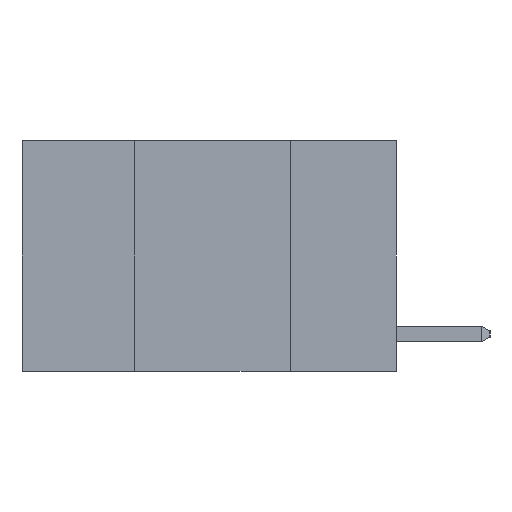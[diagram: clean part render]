
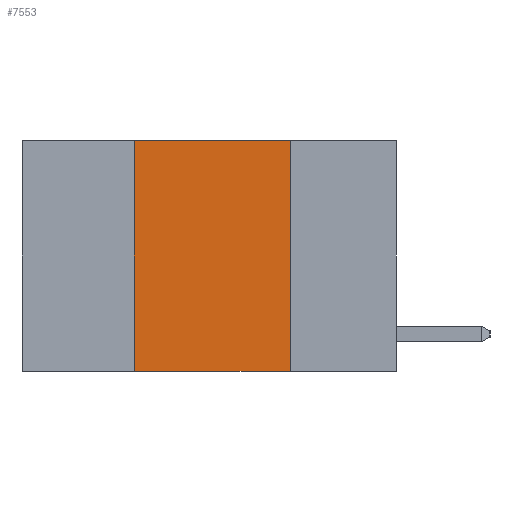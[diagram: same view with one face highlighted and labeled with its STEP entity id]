
A CAD part, left-side view. The second image highlights one B-rep face of the part: STEP entity #7553.
In plain terms, the highlighted planar face has unit normal (-1, 0, 0).
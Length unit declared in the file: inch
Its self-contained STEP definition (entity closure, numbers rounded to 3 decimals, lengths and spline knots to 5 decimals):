
#228 = VECTOR ( 'NONE', #649, 39.37008 ) ;
#649 = DIRECTION ( 'NONE',  ( 0., 0., -1. ) ) ;
#696 = DIRECTION ( 'NONE',  ( 0., 0., 1. ) ) ;
#790 = CARTESIAN_POINT ( 'NONE',  ( 0., 0.42, -0.37 ) ) ;
#941 = ORIENTED_EDGE ( 'NONE', *, *, #4402, .F. ) ;
#1168 = ORIENTED_EDGE ( 'NONE', *, *, #5838, .T. ) ;
#1659 = DIRECTION ( 'NONE',  ( 1., 0., 0. ) ) ;
#1970 = VERTEX_POINT ( 'NONE', #790 ) ;
#2298 = CARTESIAN_POINT ( 'NONE',  ( 0., 0.6, 0. ) ) ;
#2876 = ORIENTED_EDGE ( 'NONE', *, *, #8790, .F. ) ;
#2977 = DIRECTION ( 'NONE',  ( 0., -1., 0. ) ) ;
#3306 = CARTESIAN_POINT ( 'NONE',  ( 0., 0.42, 0. ) ) ;
#3360 = CARTESIAN_POINT ( 'NONE',  ( 0., 0.6, -0.37 ) ) ;
#3532 = CARTESIAN_POINT ( 'NONE',  ( 0., 0.17, 0. ) ) ;
#3566 = CARTESIAN_POINT ( 'NONE',  ( 0., 0.17, 0. ) ) ;
#3601 = VERTEX_POINT ( 'NONE', #3306 ) ;
#3860 = AXIS2_PLACEMENT_3D ( 'NONE', #5247, #1659, #6665 ) ;
#4402 = EDGE_CURVE ( 'NONE', #6031, #7622, #7837, .T. ) ;
#4522 = PLANE ( 'NONE',  #3860 ) ;
#4863 = EDGE_CURVE ( 'NONE', #1970, #3601, #8995, .T. ) ;
#5247 = CARTESIAN_POINT ( 'NONE',  ( 0., 0.6, 0. ) ) ;
#5514 = DIRECTION ( 'NONE',  ( 0., -1., 0. ) ) ;
#5838 = EDGE_CURVE ( 'NONE', #1970, #7622, #7382, .T. ) ;
#6031 = VERTEX_POINT ( 'NONE', #3532 ) ;
#6161 = FACE_OUTER_BOUND ( 'NONE', #8746, .T. ) ;
#6665 = DIRECTION ( 'NONE',  ( 0., 0., -1. ) ) ;
#6733 = CARTESIAN_POINT ( 'NONE',  ( 0., 0.17, -0.37 ) ) ;
#6994 = LINE ( 'NONE', #2298, #8618 ) ;
#7150 = CARTESIAN_POINT ( 'NONE',  ( 0., 0.42, 0. ) ) ;
#7166 = VECTOR ( 'NONE', #5514, 39.37008 ) ;
#7382 = LINE ( 'NONE', #3360, #7166 ) ;
#7397 = VECTOR ( 'NONE', #696, 39.37008 ) ;
#7553 = ADVANCED_FACE ( 'NONE', ( #6161 ), #4522, .F. ) ;
#7622 = VERTEX_POINT ( 'NONE', #6733 ) ;
#7837 = LINE ( 'NONE', #3566, #228 ) ;
#8501 = ORIENTED_EDGE ( 'NONE', *, *, #4863, .F. ) ;
#8618 = VECTOR ( 'NONE', #2977, 39.37008 ) ;
#8746 = EDGE_LOOP ( 'NONE', ( #941, #2876, #8501, #1168 ) ) ;
#8790 = EDGE_CURVE ( 'NONE', #3601, #6031, #6994, .T. ) ;
#8995 = LINE ( 'NONE', #7150, #7397 ) ;
